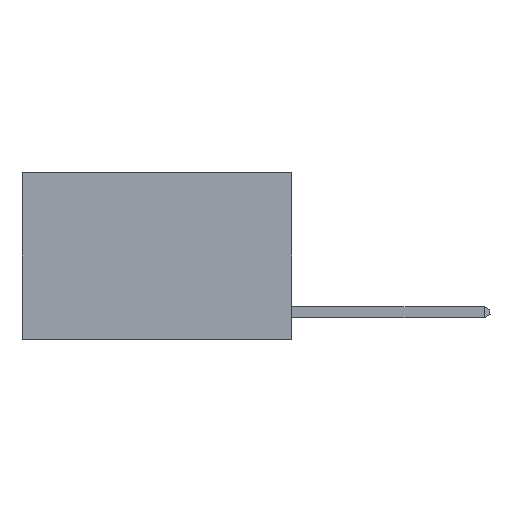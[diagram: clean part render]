
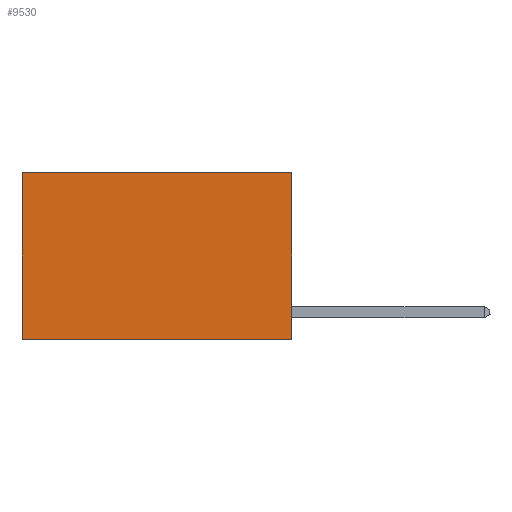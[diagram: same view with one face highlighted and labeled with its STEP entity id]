
A CAD part, left-side view. The second image highlights one B-rep face of the part: STEP entity #9530.
In plain terms, the highlighted planar face has unit normal (-1, 0, 0).
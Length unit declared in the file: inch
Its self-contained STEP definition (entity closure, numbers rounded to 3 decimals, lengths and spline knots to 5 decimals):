
#492 = DIRECTION ( 'NONE',  ( 0., 0., -1. ) ) ;
#2309 = VECTOR ( 'NONE', #20645, 39.37008 ) ;
#2547 = VECTOR ( 'NONE', #9022, 39.37008 ) ;
#5306 = EDGE_CURVE ( 'NONE', #20932, #9553, #14223, .T. ) ;
#5781 = VECTOR ( 'NONE', #18444, 39.37008 ) ;
#7202 = CARTESIAN_POINT ( 'NONE',  ( 0.2625, 0., -0.37 ) ) ;
#7859 = CARTESIAN_POINT ( 'NONE',  ( 0.2625, 0.6, 0. ) ) ;
#8639 = PLANE ( 'NONE',  #18746 ) ;
#9022 = DIRECTION ( 'NONE',  ( 0., 1., 0. ) ) ;
#9172 = LINE ( 'NONE', #20613, #12919 ) ;
#9530 = ADVANCED_FACE ( 'NONE', ( #14951 ), #8639, .F. ) ;
#9547 = VERTEX_POINT ( 'NONE', #11903 ) ;
#9553 = VERTEX_POINT ( 'NONE', #18257 ) ;
#10222 = CARTESIAN_POINT ( 'NONE',  ( 0.2625, 0.6, 0. ) ) ;
#10263 = DIRECTION ( 'NONE',  ( 1., 0., 0. ) ) ;
#10612 = LINE ( 'NONE', #7202, #5781 ) ;
#10708 = LINE ( 'NONE', #15428, #2547 ) ;
#11614 = ORIENTED_EDGE ( 'NONE', *, *, #14217, .T. ) ;
#11903 = CARTESIAN_POINT ( 'NONE',  ( 0.2625, 0., 0. ) ) ;
#12919 = VECTOR ( 'NONE', #14224, 39.37008 ) ;
#13214 = VERTEX_POINT ( 'NONE', #19380 ) ;
#14217 = EDGE_CURVE ( 'NONE', #9547, #20932, #10708, .T. ) ;
#14223 = LINE ( 'NONE', #7859, #2309 ) ;
#14224 = DIRECTION ( 'NONE',  ( 0., 0., -1. ) ) ;
#14951 = FACE_OUTER_BOUND ( 'NONE', #16817, .T. ) ;
#15428 = CARTESIAN_POINT ( 'NONE',  ( 0.2625, 0., 0. ) ) ;
#15993 = ORIENTED_EDGE ( 'NONE', *, *, #17959, .F. ) ;
#16020 = ORIENTED_EDGE ( 'NONE', *, *, #5306, .T. ) ;
#16314 = EDGE_CURVE ( 'NONE', #9547, #13214, #9172, .T. ) ;
#16508 = ORIENTED_EDGE ( 'NONE', *, *, #16314, .F. ) ;
#16817 = EDGE_LOOP ( 'NONE', ( #16020, #15993, #16508, #11614 ) ) ;
#17959 = EDGE_CURVE ( 'NONE', #13214, #9553, #10612, .T. ) ;
#18257 = CARTESIAN_POINT ( 'NONE',  ( 0.2625, 0.6, -0.37 ) ) ;
#18444 = DIRECTION ( 'NONE',  ( 0., 1., 0. ) ) ;
#18746 = AXIS2_PLACEMENT_3D ( 'NONE', #19864, #10263, #492 ) ;
#19380 = CARTESIAN_POINT ( 'NONE',  ( 0.2625, 0., -0.37 ) ) ;
#19864 = CARTESIAN_POINT ( 'NONE',  ( 0.2625, 0., 0. ) ) ;
#20613 = CARTESIAN_POINT ( 'NONE',  ( 0.2625, 0., 0. ) ) ;
#20645 = DIRECTION ( 'NONE',  ( 0., 0., -1. ) ) ;
#20932 = VERTEX_POINT ( 'NONE', #10222 ) ;
